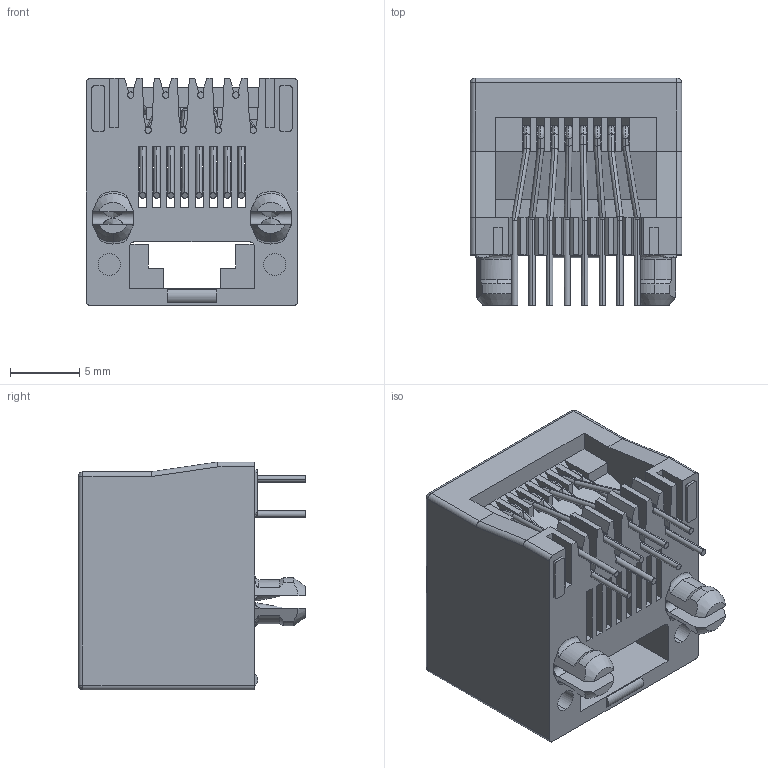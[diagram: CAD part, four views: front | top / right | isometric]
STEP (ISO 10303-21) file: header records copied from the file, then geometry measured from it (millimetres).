
FILE_DESCRIPTION (( 'STEP AP203' ), '1' );
FILE_NAME ('RJ28018821P00031.STEP', '2020-01-15T16:45:03', ( '' ), ( '' ), 'SwSTEP 2.0', 'SolidWorks 2016', '' );
FILE_SCHEMA (( 'CONFIG_CONTROL_DESIGN' ));
Length unit declared in the file: millimetre
Products named in the file (3): RJ28018821P00031; 28 Contacts; 28 Insulator
Assembly tree (2 placements, depth 2):
  RJ28018821P00031
    28 Insulator
    28 Contacts
Bounding box: 15.3 x 16.5 x 16.5 mm (x, y, z)
Volume: 1535.1 mm3; surface area: 2745.5 mm2
Topology: 9 solids, 9 shells, 580 faces, 1649 edges, 1065 vertices
Faces by surface type: plane 319, cylinder 205, bspline 44, cone 12
Entity records: 21399 total; most frequent: CARTESIAN_POINT 6573, ORIENTED_EDGE 3290, DIRECTION 2717, EDGE_CURVE 1645, VERTEX_POINT 1065, LINE 1047, VECTOR 1047, AXIS2_PLACEMENT_3D 835
